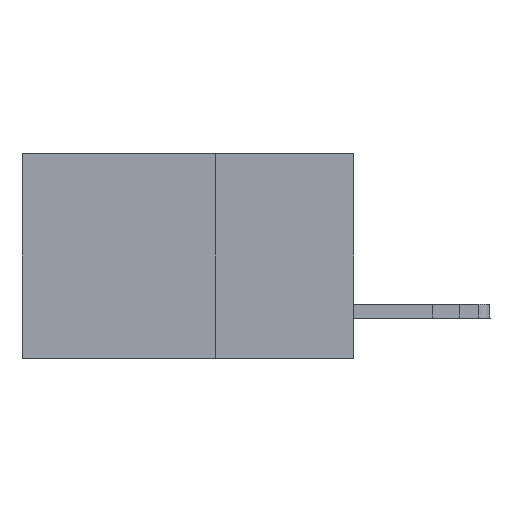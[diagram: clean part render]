
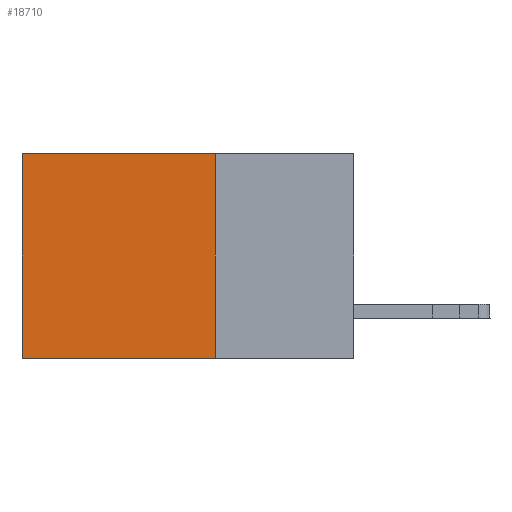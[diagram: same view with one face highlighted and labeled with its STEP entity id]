
A CAD part, left-side view. The second image highlights one B-rep face of the part: STEP entity #18710.
In plain terms, the highlighted planar face has unit normal (-1, 0, 0).
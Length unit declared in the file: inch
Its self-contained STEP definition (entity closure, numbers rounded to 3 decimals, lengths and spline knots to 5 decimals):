
#467 = AXIS2_PLACEMENT_3D ( 'NONE', #20023, #22152, #9781 ) ;
#937 = LINE ( 'NONE', #14663, #6454 ) ;
#1373 = CARTESIAN_POINT ( 'NONE',  ( 0.2875, 0.6, 0. ) ) ;
#1540 = VERTEX_POINT ( 'NONE', #11949 ) ;
#2052 = VECTOR ( 'NONE', #12152, 39.37008 ) ;
#2239 = VECTOR ( 'NONE', #10381, 39.37008 ) ;
#3131 = PLANE ( 'NONE',  #467 ) ;
#4877 = EDGE_CURVE ( 'NONE', #1540, #20693, #16177, .T. ) ;
#5268 = ORIENTED_EDGE ( 'NONE', *, *, #9754, .F. ) ;
#5845 = CARTESIAN_POINT ( 'NONE',  ( 0.2875, 0.25, 0. ) ) ;
#6454 = VECTOR ( 'NONE', #21519, 39.37008 ) ;
#6638 = VERTEX_POINT ( 'NONE', #11531 ) ;
#8527 = EDGE_CURVE ( 'NONE', #20693, #19621, #13742, .T. ) ;
#9754 = EDGE_CURVE ( 'NONE', #1540, #6638, #937, .T. ) ;
#9781 = DIRECTION ( 'NONE',  ( 0., 0., -1. ) ) ;
#10381 = DIRECTION ( 'NONE',  ( 0., 0., -1. ) ) ;
#11118 = ORIENTED_EDGE ( 'NONE', *, *, #8527, .T. ) ;
#11440 = ORIENTED_EDGE ( 'NONE', *, *, #21328, .F. ) ;
#11531 = CARTESIAN_POINT ( 'NONE',  ( 0.2875, 0.25, -0.37 ) ) ;
#11810 = FACE_OUTER_BOUND ( 'NONE', #15015, .T. ) ;
#11949 = CARTESIAN_POINT ( 'NONE',  ( 0.2875, 0.25, 0. ) ) ;
#12152 = DIRECTION ( 'NONE',  ( 0., 1., 0. ) ) ;
#12695 = DIRECTION ( 'NONE',  ( 0., 1., 0. ) ) ;
#13193 = CARTESIAN_POINT ( 'NONE',  ( 0.2875, 0.6, 0. ) ) ;
#13742 = LINE ( 'NONE', #1373, #2239 ) ;
#14152 = LINE ( 'NONE', #19010, #2052 ) ;
#14663 = CARTESIAN_POINT ( 'NONE',  ( 0.2875, 0.25, 0. ) ) ;
#15015 = EDGE_LOOP ( 'NONE', ( #11118, #11440, #5268, #16801 ) ) ;
#16177 = LINE ( 'NONE', #5845, #19606 ) ;
#16801 = ORIENTED_EDGE ( 'NONE', *, *, #4877, .T. ) ;
#18710 = ADVANCED_FACE ( 'NONE', ( #11810 ), #3131, .F. ) ;
#19010 = CARTESIAN_POINT ( 'NONE',  ( 0.2875, 0.25, -0.37 ) ) ;
#19606 = VECTOR ( 'NONE', #12695, 39.37008 ) ;
#19621 = VERTEX_POINT ( 'NONE', #21537 ) ;
#20023 = CARTESIAN_POINT ( 'NONE',  ( 0.2875, 0.25, 0. ) ) ;
#20693 = VERTEX_POINT ( 'NONE', #13193 ) ;
#21328 = EDGE_CURVE ( 'NONE', #6638, #19621, #14152, .T. ) ;
#21519 = DIRECTION ( 'NONE',  ( 0., 0., -1. ) ) ;
#21537 = CARTESIAN_POINT ( 'NONE',  ( 0.2875, 0.6, -0.37 ) ) ;
#22152 = DIRECTION ( 'NONE',  ( 1., 0., 0. ) ) ;
